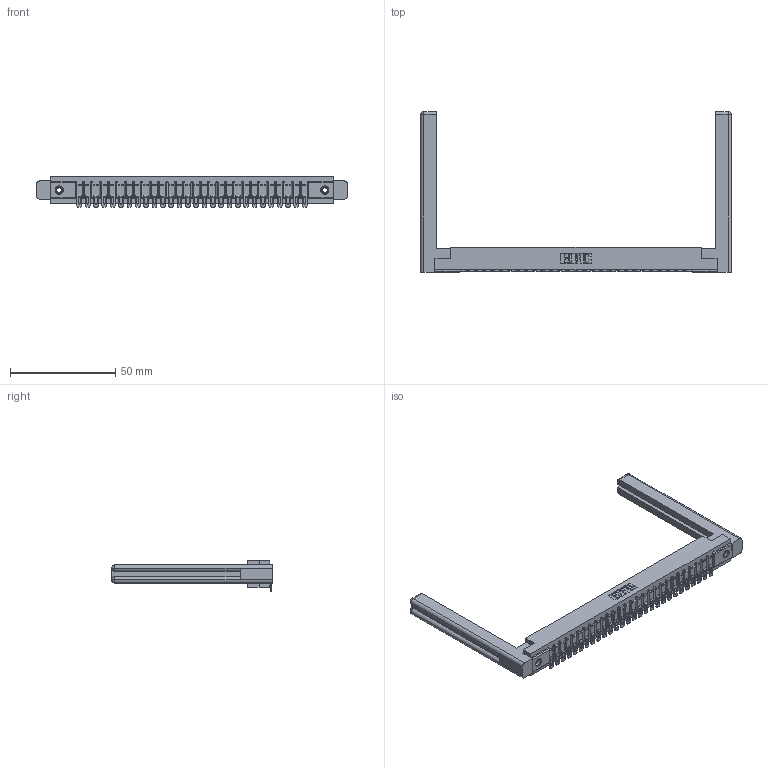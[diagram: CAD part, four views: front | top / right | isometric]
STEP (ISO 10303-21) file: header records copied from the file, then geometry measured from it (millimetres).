
FILE_DESCRIPTION (( 'STEP AP203' ), '1' );
FILE_NAME ('307-028-454-158.STEP', '2020-09-28T07:54:17', ( '' ), ( '' ), 'SwSTEP 2.0', 'SolidWorks 2020', '' );
FILE_SCHEMA (( 'CONFIG_CONTROL_DESIGN' ));
Length unit declared in the file: inch
Products named in the file (5): 345-250-001_345-250-001-102; 307-028-454-158; 307-290-002_554; 307-220-058; 307 Part_.156 Dia Mounting Holes
Assembly tree (33 placements, depth 2):
  307-028-454-158
    307 Part_.156 Dia Mounting Holes
    307-290-002_554  x28
    307-220-058  x2
    345-250-001_345-250-001-102  x2
Bounding box: 147.57 x 76.33 x 14.52 mm (x, y, z)
Volume: 22818.2 mm3; surface area: 24371.2 mm2
Topology: 33 solids, 33 shells, 2557 faces, 7761 edges, 5082 vertices
Faces by surface type: plane 1442, cylinder 1033, sphere 58, torus 12, cone 12
Entity records: 29328 total; most frequent: CARTESIAN_POINT 4953, ORIENTED_EDGE 4882, DIRECTION 4785, EDGE_CURVE 2441, VECTOR 1853, LINE 1853, VERTEX_POINT 1580, AXIS2_PLACEMENT_3D 1466
